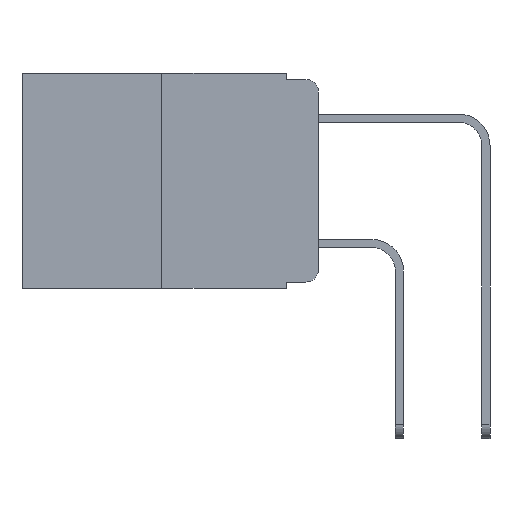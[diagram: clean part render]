
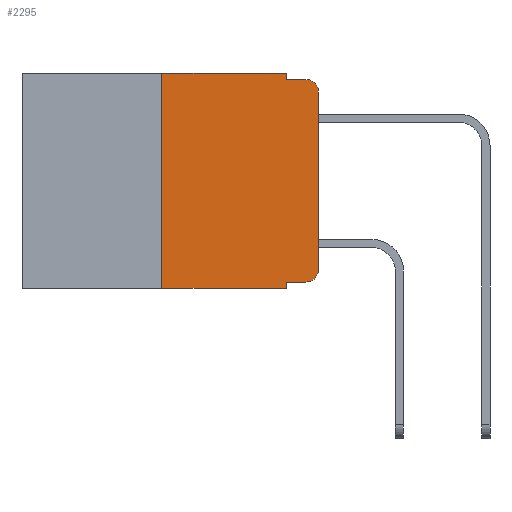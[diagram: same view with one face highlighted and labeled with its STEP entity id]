
A CAD part, left-side view. The second image highlights one B-rep face of the part: STEP entity #2295.
In plain terms, the highlighted planar face has unit normal (-1, 0, 0).
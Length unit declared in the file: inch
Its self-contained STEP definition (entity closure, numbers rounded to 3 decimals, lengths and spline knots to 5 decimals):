
#234 = CARTESIAN_POINT ( 'NONE',  ( 0., 0.02, -0.01 ) ) ;
#244 = DIRECTION ( 'NONE',  ( 0., -1., 0. ) ) ;
#245 = CIRCLE ( 'NONE', #1801, 0.02 ) ;
#699 = VECTOR ( 'NONE', #4285, 39.37008 ) ;
#752 = EDGE_CURVE ( 'NONE', #2402, #5560, #8855, .T. ) ;
#883 = EDGE_CURVE ( 'NONE', #8536, #10696, #5644, .T. ) ;
#1072 = ORIENTED_EDGE ( 'NONE', *, *, #12064, .F. ) ;
#1801 = AXIS2_PLACEMENT_3D ( 'NONE', #9731, #3803, #10651 ) ;
#1834 = DIRECTION ( 'NONE',  ( 0., -1., 0. ) ) ;
#2112 = LINE ( 'NONE', #7838, #12161 ) ;
#2177 = LINE ( 'NONE', #11623, #12208 ) ;
#2295 = ADVANCED_FACE ( 'NONE', ( #10998 ), #9111, .F. ) ;
#2402 = VERTEX_POINT ( 'NONE', #3787 ) ;
#2420 = VECTOR ( 'NONE', #6682, 39.37008 ) ;
#2422 = ORIENTED_EDGE ( 'NONE', *, *, #883, .F. ) ;
#2437 = ORIENTED_EDGE ( 'NONE', *, *, #752, .T. ) ;
#2476 = ORIENTED_EDGE ( 'NONE', *, *, #11757, .F. ) ;
#2571 = ORIENTED_EDGE ( 'NONE', *, *, #5693, .T. ) ;
#2705 = CARTESIAN_POINT ( 'NONE',  ( 0., 0.25, -0.343 ) ) ;
#3254 = CARTESIAN_POINT ( 'NONE',  ( 0., 0., 0. ) ) ;
#3380 = EDGE_LOOP ( 'NONE', ( #9947, #2571, #2476, #2422, #10087, #1072, #4557, #7524, #2437, #5834 ) ) ;
#3646 = CARTESIAN_POINT ( 'NONE',  ( 0., 0.051, 0. ) ) ;
#3787 = CARTESIAN_POINT ( 'NONE',  ( 0., 0.051, -0.333 ) ) ;
#3803 = DIRECTION ( 'NONE',  ( -1., 0., 0. ) ) ;
#3840 = CARTESIAN_POINT ( 'NONE',  ( 0., 0.25, 0. ) ) ;
#3851 = EDGE_CURVE ( 'NONE', #12534, #8536, #2112, .T. ) ;
#3886 = VECTOR ( 'NONE', #244, 39.37008 ) ;
#4208 = CIRCLE ( 'NONE', #7439, 0.02 ) ;
#4285 = DIRECTION ( 'NONE',  ( 0., -1., 0. ) ) ;
#4307 = DIRECTION ( 'NONE',  ( 0., 0., 1. ) ) ;
#4509 = CARTESIAN_POINT ( 'NONE',  ( 0., 0., -0.313 ) ) ;
#4557 = ORIENTED_EDGE ( 'NONE', *, *, #8284, .T. ) ;
#5105 = DIRECTION ( 'NONE',  ( 0., 0., 1. ) ) ;
#5115 = CARTESIAN_POINT ( 'NONE',  ( 0., 0.051, -0.343 ) ) ;
#5157 = VECTOR ( 'NONE', #5105, 39.37008 ) ;
#5158 = CARTESIAN_POINT ( 'NONE',  ( 0., 0.051, -0.01 ) ) ;
#5185 = LINE ( 'NONE', #3646, #2420 ) ;
#5304 = VECTOR ( 'NONE', #4307, 39.37008 ) ;
#5473 = DIRECTION ( 'NONE',  ( -1., 0., 0. ) ) ;
#5560 = VERTEX_POINT ( 'NONE', #9108 ) ;
#5644 = LINE ( 'NONE', #12180, #12517 ) ;
#5693 = EDGE_CURVE ( 'NONE', #8163, #9246, #4208, .T. ) ;
#5834 = ORIENTED_EDGE ( 'NONE', *, *, #9430, .T. ) ;
#5996 = DIRECTION ( 'NONE',  ( 0., -1., 0. ) ) ;
#6023 = DIRECTION ( 'NONE',  ( 1., 0., 0. ) ) ;
#6336 = AXIS2_PLACEMENT_3D ( 'NONE', #9454, #6023, #7014 ) ;
#6563 = LINE ( 'NONE', #8426, #3886 ) ;
#6682 = DIRECTION ( 'NONE',  ( 0., 0., -1. ) ) ;
#7014 = DIRECTION ( 'NONE',  ( 0., 0., -1. ) ) ;
#7434 = EDGE_CURVE ( 'NONE', #12309, #8163, #10454, .T. ) ;
#7439 = AXIS2_PLACEMENT_3D ( 'NONE', #11180, #5473, #12060 ) ;
#7524 = ORIENTED_EDGE ( 'NONE', *, *, #11261, .F. ) ;
#7838 = CARTESIAN_POINT ( 'NONE',  ( 0., 0.473, 0. ) ) ;
#8163 = VERTEX_POINT ( 'NONE', #10597 ) ;
#8284 = EDGE_CURVE ( 'NONE', #9435, #10693, #2177, .T. ) ;
#8426 = CARTESIAN_POINT ( 'NONE',  ( 0., 0.051, -0.01 ) ) ;
#8536 = VERTEX_POINT ( 'NONE', #10195 ) ;
#8606 = CARTESIAN_POINT ( 'NONE',  ( 0., 0.051, -0.333 ) ) ;
#8855 = LINE ( 'NONE', #8606, #699 ) ;
#9108 = CARTESIAN_POINT ( 'NONE',  ( 0., 0.02, -0.333 ) ) ;
#9111 = PLANE ( 'NONE',  #6336 ) ;
#9246 = VERTEX_POINT ( 'NONE', #234 ) ;
#9430 = EDGE_CURVE ( 'NONE', #5560, #12309, #245, .T. ) ;
#9435 = VERTEX_POINT ( 'NONE', #2705 ) ;
#9454 = CARTESIAN_POINT ( 'NONE',  ( 0., 0.473, 0. ) ) ;
#9731 = CARTESIAN_POINT ( 'NONE',  ( 0., 0.02, -0.313 ) ) ;
#9947 = ORIENTED_EDGE ( 'NONE', *, *, #7434, .T. ) ;
#10087 = ORIENTED_EDGE ( 'NONE', *, *, #3851, .F. ) ;
#10195 = CARTESIAN_POINT ( 'NONE',  ( 0., 0.051, 0. ) ) ;
#10454 = LINE ( 'NONE', #3254, #5304 ) ;
#10597 = CARTESIAN_POINT ( 'NONE',  ( 0., 0., -0.03 ) ) ;
#10651 = DIRECTION ( 'NONE',  ( 0., 0., -1. ) ) ;
#10693 = VERTEX_POINT ( 'NONE', #5115 ) ;
#10696 = VERTEX_POINT ( 'NONE', #5158 ) ;
#10736 = DIRECTION ( 'NONE',  ( 0., 0., -1. ) ) ;
#10879 = CARTESIAN_POINT ( 'NONE',  ( 0., 0.25, 0. ) ) ;
#10998 = FACE_OUTER_BOUND ( 'NONE', #3380, .T. ) ;
#11180 = CARTESIAN_POINT ( 'NONE',  ( 0., 0.02, -0.03 ) ) ;
#11261 = EDGE_CURVE ( 'NONE', #2402, #10693, #5185, .T. ) ;
#11623 = CARTESIAN_POINT ( 'NONE',  ( 0., 0.473, -0.343 ) ) ;
#11757 = EDGE_CURVE ( 'NONE', #10696, #9246, #6563, .T. ) ;
#12060 = DIRECTION ( 'NONE',  ( 0., 0., -1. ) ) ;
#12064 = EDGE_CURVE ( 'NONE', #9435, #12534, #12375, .T. ) ;
#12161 = VECTOR ( 'NONE', #5996, 39.37008 ) ;
#12180 = CARTESIAN_POINT ( 'NONE',  ( 0., 0.051, 0. ) ) ;
#12208 = VECTOR ( 'NONE', #1834, 39.37008 ) ;
#12309 = VERTEX_POINT ( 'NONE', #4509 ) ;
#12375 = LINE ( 'NONE', #10879, #5157 ) ;
#12517 = VECTOR ( 'NONE', #10736, 39.37008 ) ;
#12534 = VERTEX_POINT ( 'NONE', #3840 ) ;
